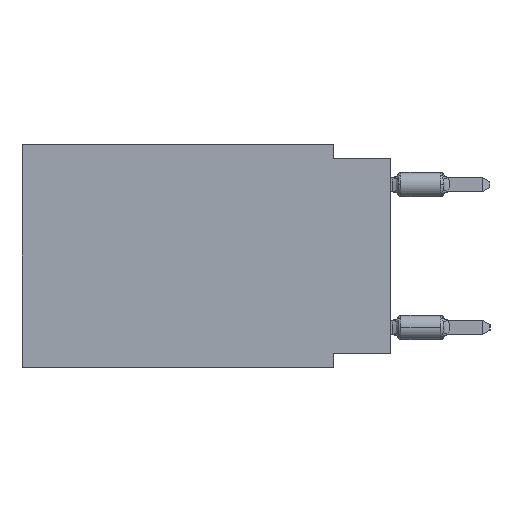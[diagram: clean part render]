
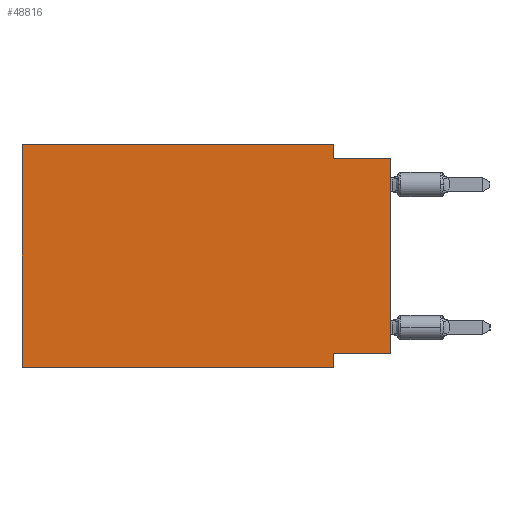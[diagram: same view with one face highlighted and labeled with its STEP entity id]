
A CAD part, left-side view. The second image highlights one B-rep face of the part: STEP entity #48816.
In plain terms, the highlighted planar face has unit normal (-1, 0, 0).
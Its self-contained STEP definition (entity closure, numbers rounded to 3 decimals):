
#118 = VECTOR ( 'NONE', #20298, 1000. ) ;
#300 = LINE ( 'NONE', #8020, #23908 ) ;
#1141 = VERTEX_POINT ( 'NONE', #29196 ) ;
#1638 = CARTESIAN_POINT ( 'NONE',  ( 0., 2.54, -9.906 ) ) ;
#1732 = EDGE_CURVE ( 'NONE', #39528, #1141, #19269, .T. ) ;
#2363 = EDGE_CURVE ( 'NONE', #30756, #4405, #37238, .T. ) ;
#2887 = EDGE_CURVE ( 'NONE', #4405, #27354, #3607, .T. ) ;
#3607 = LINE ( 'NONE', #14709, #33149 ) ;
#4405 = VERTEX_POINT ( 'NONE', #12365 ) ;
#6250 = DIRECTION ( 'NONE',  ( 0., -1., 0. ) ) ;
#8020 = CARTESIAN_POINT ( 'NONE',  ( 0., 16.383, 0. ) ) ;
#8498 = EDGE_LOOP ( 'NONE', ( #35501, #39398, #38963, #33488, #9875, #16956, #45678, #25257 ) ) ;
#8713 = CARTESIAN_POINT ( 'NONE',  ( 0., 16.383, 0. ) ) ;
#9141 = CARTESIAN_POINT ( 'NONE',  ( 0., 0., -9.271 ) ) ;
#9875 = ORIENTED_EDGE ( 'NONE', *, *, #17003, .F. ) ;
#10594 = VERTEX_POINT ( 'NONE', #28398 ) ;
#11948 = CARTESIAN_POINT ( 'NONE',  ( 0., 2.54, -9.271 ) ) ;
#12365 = CARTESIAN_POINT ( 'NONE',  ( 0., 2.54, 0. ) ) ;
#13710 = DIRECTION ( 'NONE',  ( 0., 1., 0. ) ) ;
#14709 = CARTESIAN_POINT ( 'NONE',  ( 0., 2.54, 0. ) ) ;
#16331 = LINE ( 'NONE', #33336, #22647 ) ;
#16364 = DIRECTION ( 'NONE',  ( 0., 0., -1. ) ) ;
#16938 = LINE ( 'NONE', #28794, #33732 ) ;
#16956 = ORIENTED_EDGE ( 'NONE', *, *, #43142, .T. ) ;
#17003 = EDGE_CURVE ( 'NONE', #18265, #30756, #300, .T. ) ;
#18265 = VERTEX_POINT ( 'NONE', #39817 ) ;
#19269 = LINE ( 'NONE', #43524, #118 ) ;
#19582 = CARTESIAN_POINT ( 'NONE',  ( 0., 16.383, -9.906 ) ) ;
#20298 = DIRECTION ( 'NONE',  ( 0., 0., 1. ) ) ;
#20596 = FACE_OUTER_BOUND ( 'NONE', #8498, .T. ) ;
#22647 = VECTOR ( 'NONE', #13710, 1000. ) ;
#23908 = VECTOR ( 'NONE', #38987, 1000. ) ;
#24110 = EDGE_CURVE ( 'NONE', #39528, #42766, #16331, .T. ) ;
#25257 = ORIENTED_EDGE ( 'NONE', *, *, #24110, .F. ) ;
#26085 = VECTOR ( 'NONE', #43835, 1000. ) ;
#26833 = DIRECTION ( 'NONE',  ( 0., 0., -1. ) ) ;
#27354 = VERTEX_POINT ( 'NONE', #33638 ) ;
#28398 = CARTESIAN_POINT ( 'NONE',  ( 0., 2.54, -9.906 ) ) ;
#28794 = CARTESIAN_POINT ( 'NONE',  ( 0., 0., -0.635 ) ) ;
#29196 = CARTESIAN_POINT ( 'NONE',  ( 0., 0., -0.635 ) ) ;
#30641 = VECTOR ( 'NONE', #6250, 1000. ) ;
#30756 = VERTEX_POINT ( 'NONE', #35849 ) ;
#32708 = PLANE ( 'NONE',  #45294 ) ;
#32856 = EDGE_CURVE ( 'NONE', #42766, #10594, #40101, .T. ) ;
#32966 = DIRECTION ( 'NONE',  ( 0., 0., -1. ) ) ;
#33056 = VECTOR ( 'NONE', #16364, 1000. ) ;
#33149 = VECTOR ( 'NONE', #26833, 1000. ) ;
#33336 = CARTESIAN_POINT ( 'NONE',  ( 0., 0., -9.271 ) ) ;
#33488 = ORIENTED_EDGE ( 'NONE', *, *, #2363, .F. ) ;
#33638 = CARTESIAN_POINT ( 'NONE',  ( 0., 2.54, -0.635 ) ) ;
#33732 = VECTOR ( 'NONE', #36303, 1000. ) ;
#35501 = ORIENTED_EDGE ( 'NONE', *, *, #1732, .T. ) ;
#35849 = CARTESIAN_POINT ( 'NONE',  ( 0., 16.383, 0. ) ) ;
#36303 = DIRECTION ( 'NONE',  ( 0., -1., 0. ) ) ;
#37238 = LINE ( 'NONE', #49868, #30641 ) ;
#38963 = ORIENTED_EDGE ( 'NONE', *, *, #2887, .F. ) ;
#38987 = DIRECTION ( 'NONE',  ( 0., 0., 1. ) ) ;
#39398 = ORIENTED_EDGE ( 'NONE', *, *, #46422, .F. ) ;
#39528 = VERTEX_POINT ( 'NONE', #9141 ) ;
#39817 = CARTESIAN_POINT ( 'NONE',  ( 0., 16.383, -9.906 ) ) ;
#40101 = LINE ( 'NONE', #1638, #33056 ) ;
#42766 = VERTEX_POINT ( 'NONE', #11948 ) ;
#43142 = EDGE_CURVE ( 'NONE', #18265, #10594, #47185, .T. ) ;
#43524 = CARTESIAN_POINT ( 'NONE',  ( 0., 0., 0. ) ) ;
#43835 = DIRECTION ( 'NONE',  ( 0., -1., 0. ) ) ;
#45294 = AXIS2_PLACEMENT_3D ( 'NONE', #8713, #48206, #32966 ) ;
#45678 = ORIENTED_EDGE ( 'NONE', *, *, #32856, .F. ) ;
#46422 = EDGE_CURVE ( 'NONE', #27354, #1141, #16938, .T. ) ;
#47185 = LINE ( 'NONE', #19582, #26085 ) ;
#48206 = DIRECTION ( 'NONE',  ( 1., 0., 0. ) ) ;
#48816 = ADVANCED_FACE ( 'NONE', ( #20596 ), #32708, .F. ) ;
#49868 = CARTESIAN_POINT ( 'NONE',  ( 0., 16.383, 0. ) ) ;
